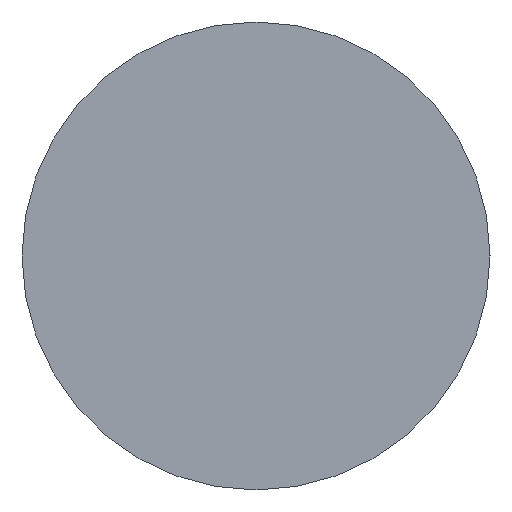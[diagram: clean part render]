
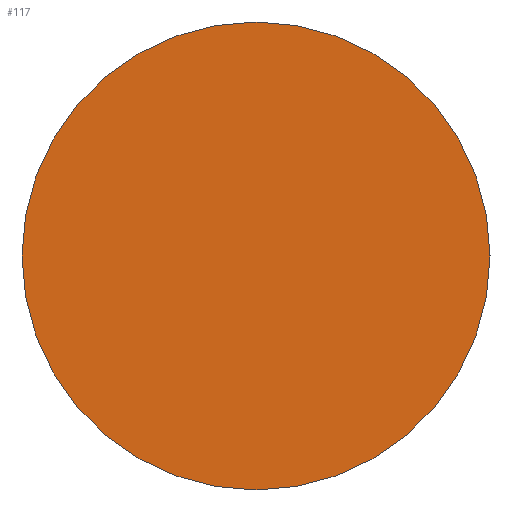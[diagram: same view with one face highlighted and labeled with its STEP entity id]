
A CAD part, left-side view. The second image highlights one B-rep face of the part: STEP entity #117.
In plain terms, the highlighted planar face has unit normal (-1, 0, 0).
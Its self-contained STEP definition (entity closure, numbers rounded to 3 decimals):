
#7 = CIRCLE ( 'NONE', #161, 5. ) ;
#10 = AXIS2_PLACEMENT_3D ( 'NONE', #99, #77, #87 ) ;
#12 = DIRECTION ( 'NONE',  ( 0., 0., -1. ) ) ;
#14 = DIRECTION ( 'NONE',  ( 1., 0., 0. ) ) ;
#16 = PLANE ( 'NONE',  #76 ) ;
#35 = CARTESIAN_POINT ( 'NONE',  ( 0., 0., -5. ) ) ;
#37 = CARTESIAN_POINT ( 'NONE',  ( 0., 0., 0. ) ) ;
#41 = EDGE_CURVE ( 'NONE', #60, #130, #84, .T. ) ;
#45 = EDGE_CURVE ( 'NONE', #130, #60, #7, .T. ) ;
#48 = EDGE_LOOP ( 'NONE', ( #136, #107 ) ) ;
#49 = CARTESIAN_POINT ( 'NONE',  ( 0., 0., 0. ) ) ;
#60 = VERTEX_POINT ( 'NONE', #155 ) ;
#65 = DIRECTION ( 'NONE',  ( 0., 0., -1. ) ) ;
#67 = DIRECTION ( 'NONE',  ( 1., 0., 0. ) ) ;
#76 = AXIS2_PLACEMENT_3D ( 'NONE', #37, #14, #12 ) ;
#77 = DIRECTION ( 'NONE',  ( 1., 0., 0. ) ) ;
#84 = CIRCLE ( 'NONE', #10, 5. ) ;
#87 = DIRECTION ( 'NONE',  ( 0., 0., -1. ) ) ;
#99 = CARTESIAN_POINT ( 'NONE',  ( 0., 0., 0. ) ) ;
#107 = ORIENTED_EDGE ( 'NONE', *, *, #45, .F. ) ;
#117 = ADVANCED_FACE ( 'NONE', ( #126 ), #16, .F. ) ;
#126 = FACE_OUTER_BOUND ( 'NONE', #48, .T. ) ;
#130 = VERTEX_POINT ( 'NONE', #35 ) ;
#136 = ORIENTED_EDGE ( 'NONE', *, *, #41, .F. ) ;
#155 = CARTESIAN_POINT ( 'NONE',  ( 0., 0., 5. ) ) ;
#161 = AXIS2_PLACEMENT_3D ( 'NONE', #49, #67, #65 ) ;
